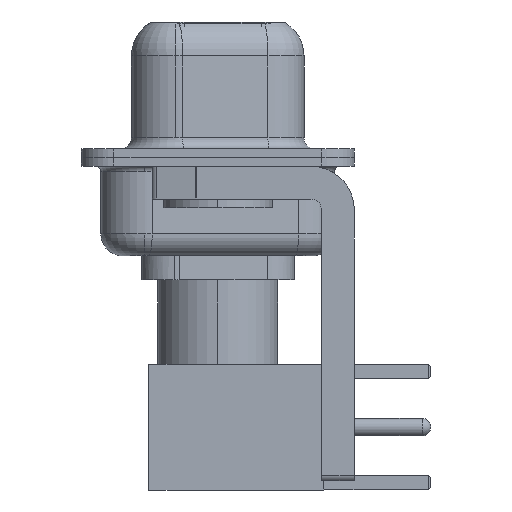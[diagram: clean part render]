
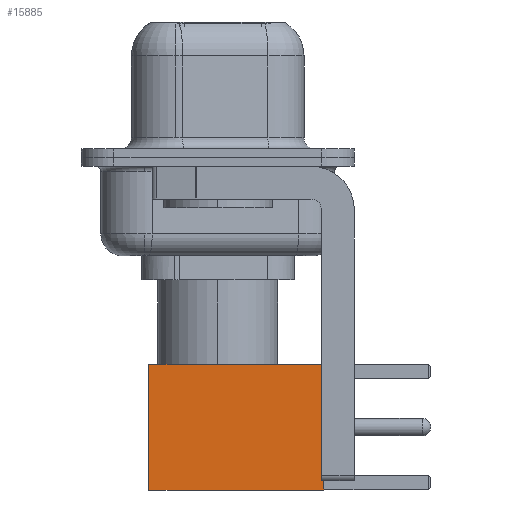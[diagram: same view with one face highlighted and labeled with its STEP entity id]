
A CAD part, left-side view. The second image highlights one B-rep face of the part: STEP entity #15885.
In plain terms, the highlighted face is planar.
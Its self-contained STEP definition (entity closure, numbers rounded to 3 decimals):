
#123 = LINE ( 'NONE', #4254, #9906 ) ;
#131 = EDGE_CURVE ( 'NONE', #7327, #16140, #10257, .T. ) ;
#133 = ORIENTED_EDGE ( 'NONE', *, *, #17152, .F. ) ;
#699 = LINE ( 'NONE', #16056, #14176 ) ;
#867 = DIRECTION ( 'NONE',  ( 0., 0., 1. ) ) ;
#1374 = DIRECTION ( 'NONE',  ( -1., 0., 0. ) ) ;
#2399 = DIRECTION ( 'NONE',  ( 0., 1., 0. ) ) ;
#2509 = EDGE_CURVE ( 'NONE', #13278, #7327, #8367, .T. ) ;
#2633 = VERTEX_POINT ( 'NONE', #12824 ) ;
#3182 = VECTOR ( 'NONE', #12115, 1000. ) ;
#3445 = DIRECTION ( 'NONE',  ( -1., 0., 0. ) ) ;
#4254 = CARTESIAN_POINT ( 'NONE',  ( 0., 2.875, 8. ) ) ;
#5092 = PLANE ( 'NONE',  #13022 ) ;
#5774 = ORIENTED_EDGE ( 'NONE', *, *, #131, .T. ) ;
#6394 = EDGE_CURVE ( 'NONE', #2633, #16140, #699, .T. ) ;
#7141 = CARTESIAN_POINT ( 'NONE',  ( 2.875, 2.875, 8. ) ) ;
#7327 = VERTEX_POINT ( 'NONE', #10644 ) ;
#7968 = EDGE_LOOP ( 'NONE', ( #10497, #5774, #15960, #133 ) ) ;
#8367 = LINE ( 'NONE', #12384, #3182 ) ;
#8915 = CARTESIAN_POINT ( 'NONE',  ( 0., 2.875, 0. ) ) ;
#9906 = VECTOR ( 'NONE', #1374, 1000. ) ;
#10257 = LINE ( 'NONE', #8915, #11115 ) ;
#10472 = DIRECTION ( 'NONE',  ( 0., 0., -1. ) ) ;
#10497 = ORIENTED_EDGE ( 'NONE', *, *, #2509, .T. ) ;
#10644 = CARTESIAN_POINT ( 'NONE',  ( 2.875, 2.875, 0. ) ) ;
#11115 = VECTOR ( 'NONE', #3445, 1000. ) ;
#12115 = DIRECTION ( 'NONE',  ( 0., 0., -1. ) ) ;
#12384 = CARTESIAN_POINT ( 'NONE',  ( 2.875, 2.875, 0. ) ) ;
#12824 = CARTESIAN_POINT ( 'NONE',  ( -2.875, 2.875, 8. ) ) ;
#13022 = AXIS2_PLACEMENT_3D ( 'NONE', #13065, #2399, #867 ) ;
#13065 = CARTESIAN_POINT ( 'NONE',  ( 2.875, 2.875, 0. ) ) ;
#13278 = VERTEX_POINT ( 'NONE', #7141 ) ;
#13685 = CARTESIAN_POINT ( 'NONE',  ( -2.875, 2.875, 0. ) ) ;
#14176 = VECTOR ( 'NONE', #10472, 1000. ) ;
#15885 = ADVANCED_FACE ( 'NONE', ( #17118 ), #5092, .T. ) ;
#15960 = ORIENTED_EDGE ( 'NONE', *, *, #6394, .F. ) ;
#16056 = CARTESIAN_POINT ( 'NONE',  ( -2.875, 2.875, 0. ) ) ;
#16140 = VERTEX_POINT ( 'NONE', #13685 ) ;
#17118 = FACE_OUTER_BOUND ( 'NONE', #7968, .T. ) ;
#17152 = EDGE_CURVE ( 'NONE', #13278, #2633, #123, .T. ) ;
